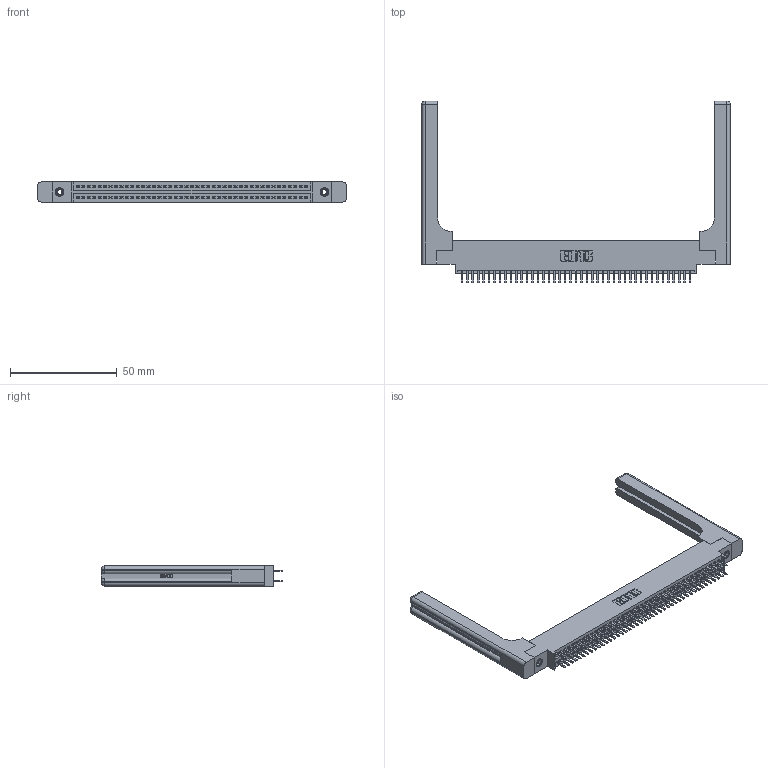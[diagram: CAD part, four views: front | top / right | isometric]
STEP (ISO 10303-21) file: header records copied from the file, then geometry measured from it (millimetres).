
FILE_DESCRIPTION (( 'STEP AP203' ), '1' );
FILE_NAME ('345-086-520-858.STEP', '2019-11-01T06:40:08', ( '' ), ( '' ), 'SwSTEP 2.0', 'SolidWorks 2016', '' );
FILE_SCHEMA (( 'CONFIG_CONTROL_DESIGN' ));
Length unit declared in the file: inch
Products named in the file (5): 345-220-058_345-220-058; 345-250-001_345-250-001-102; 345-086-520-858; 345 Part_0.170 Offset - 0.156 Dia-TH; 345-292-001_345-293-120
Assembly tree (91 placements, depth 2):
  345-086-520-858
    345 Part_0.170 Offset - 0.156 Dia-TH
    345-292-001_345-293-120  x86
    345-250-001_345-250-001-102  x2
    345-220-058_345-220-058  x2
Bounding box: 144.25 x 84.96 x 9.4 mm (x, y, z)
Volume: 22345.5 mm3; surface area: 25644 mm2
Topology: 91 solids, 91 shells, 5030 faces, 14521 edges, 9430 vertices
Faces by surface type: plane 3242, cylinder 1728, bspline 36, cone 12, sphere 8, torus 4
Entity records: 39032 total; most frequent: CARTESIAN_POINT 7549, ORIENTED_EDGE 6268, DIRECTION 5574, EDGE_CURVE 3134, VECTOR 2734, LINE 2734, VERTEX_POINT 2078, AXIS2_PLACEMENT_3D 1420
